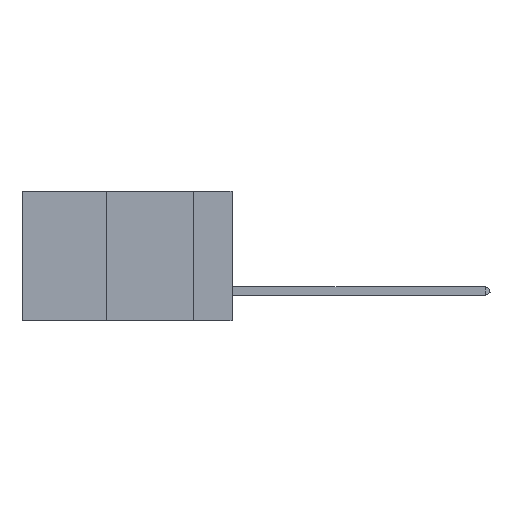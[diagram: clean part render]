
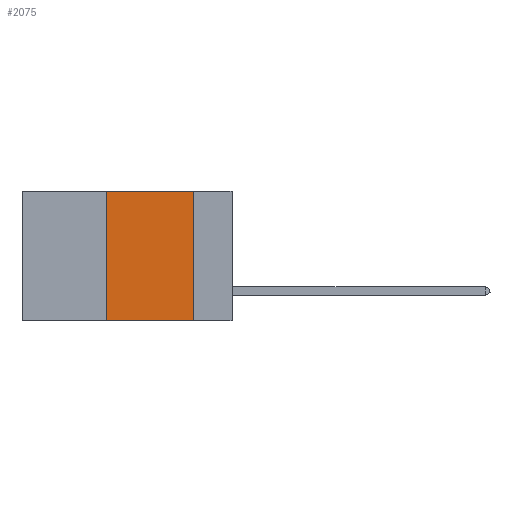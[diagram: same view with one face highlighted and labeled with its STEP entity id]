
A CAD part, left-side view. The second image highlights one B-rep face of the part: STEP entity #2075.
In plain terms, the highlighted planar face has unit normal (-1, 0, 0).
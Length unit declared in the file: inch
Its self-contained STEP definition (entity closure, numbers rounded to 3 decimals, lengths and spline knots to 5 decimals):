
#80 = LINE ( 'NONE', #9464, #4939 ) ;
#493 = LINE ( 'NONE', #6134, #3447 ) ;
#1481 = EDGE_CURVE ( 'NONE', #8978, #9619, #493, .T. ) ;
#1643 = DIRECTION ( 'NONE',  ( 0., -1., 0. ) ) ;
#1938 = ORIENTED_EDGE ( 'NONE', *, *, #1481, .T. ) ;
#2075 = ADVANCED_FACE ( 'NONE', ( #3586 ), #7125, .F. ) ;
#2113 = VERTEX_POINT ( 'NONE', #12513 ) ;
#2281 = CARTESIAN_POINT ( 'NONE',  ( 0., 0.6, 0. ) ) ;
#2321 = CARTESIAN_POINT ( 'NONE',  ( 0., 0.11, -0.37 ) ) ;
#2517 = EDGE_CURVE ( 'NONE', #8978, #2113, #6536, .T. ) ;
#3201 = DIRECTION ( 'NONE',  ( 1., 0., 0. ) ) ;
#3241 = DIRECTION ( 'NONE',  ( 0., -1., 0. ) ) ;
#3335 = ORIENTED_EDGE ( 'NONE', *, *, #2517, .F. ) ;
#3447 = VECTOR ( 'NONE', #3241, 39.37008 ) ;
#3586 = FACE_OUTER_BOUND ( 'NONE', #9324, .T. ) ;
#4159 = LINE ( 'NONE', #7739, #9048 ) ;
#4653 = EDGE_CURVE ( 'NONE', #5555, #9619, #80, .T. ) ;
#4939 = VECTOR ( 'NONE', #10840, 39.37008 ) ;
#5555 = VERTEX_POINT ( 'NONE', #9979 ) ;
#6134 = CARTESIAN_POINT ( 'NONE',  ( 0., 0.6, -0.37 ) ) ;
#6536 = LINE ( 'NONE', #10450, #7947 ) ;
#7125 = PLANE ( 'NONE',  #9828 ) ;
#7739 = CARTESIAN_POINT ( 'NONE',  ( 0., 0.6, 0. ) ) ;
#7947 = VECTOR ( 'NONE', #11436, 39.37008 ) ;
#8087 = DIRECTION ( 'NONE',  ( 0., 0., -1. ) ) ;
#8978 = VERTEX_POINT ( 'NONE', #12097 ) ;
#9048 = VECTOR ( 'NONE', #1643, 39.37008 ) ;
#9324 = EDGE_LOOP ( 'NONE', ( #12913, #9976, #3335, #1938 ) ) ;
#9464 = CARTESIAN_POINT ( 'NONE',  ( 0., 0.11, 0. ) ) ;
#9619 = VERTEX_POINT ( 'NONE', #2321 ) ;
#9828 = AXIS2_PLACEMENT_3D ( 'NONE', #2281, #3201, #8087 ) ;
#9976 = ORIENTED_EDGE ( 'NONE', *, *, #11255, .F. ) ;
#9979 = CARTESIAN_POINT ( 'NONE',  ( 0., 0.11, 0. ) ) ;
#10450 = CARTESIAN_POINT ( 'NONE',  ( 0., 0.36, 0. ) ) ;
#10840 = DIRECTION ( 'NONE',  ( 0., 0., -1. ) ) ;
#11255 = EDGE_CURVE ( 'NONE', #2113, #5555, #4159, .T. ) ;
#11436 = DIRECTION ( 'NONE',  ( 0., 0., 1. ) ) ;
#12097 = CARTESIAN_POINT ( 'NONE',  ( 0., 0.36, -0.37 ) ) ;
#12513 = CARTESIAN_POINT ( 'NONE',  ( 0., 0.36, 0. ) ) ;
#12913 = ORIENTED_EDGE ( 'NONE', *, *, #4653, .F. ) ;
